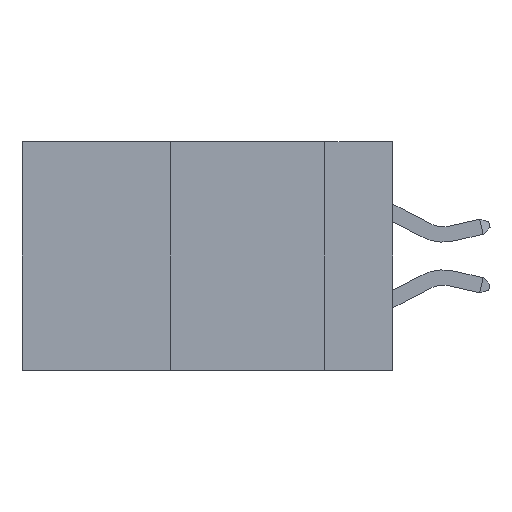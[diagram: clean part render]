
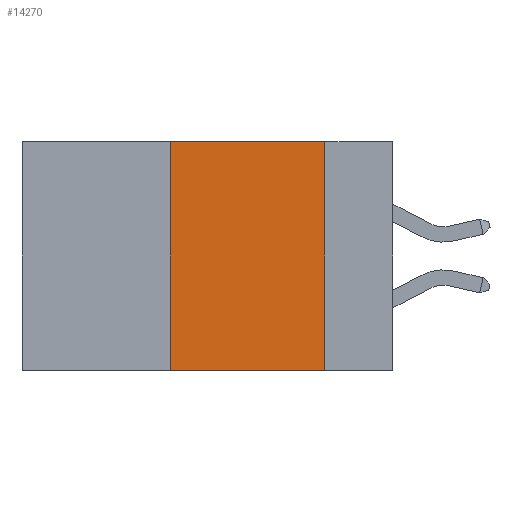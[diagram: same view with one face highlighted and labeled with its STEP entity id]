
A CAD part, left-side view. The second image highlights one B-rep face of the part: STEP entity #14270.
In plain terms, the highlighted planar face has unit normal (-1, 0, 0).
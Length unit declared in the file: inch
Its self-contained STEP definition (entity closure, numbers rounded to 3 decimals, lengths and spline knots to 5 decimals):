
#247 = VERTEX_POINT ( 'NONE', #5593 ) ;
#382 = EDGE_LOOP ( 'NONE', ( #7832, #5539, #2883, #7250 ) ) ;
#645 = EDGE_CURVE ( 'NONE', #9239, #247, #11401, .T. ) ;
#1869 = VECTOR ( 'NONE', #12145, 39.37008 ) ;
#1916 = CARTESIAN_POINT ( 'NONE',  ( 0., 0.6, 0. ) ) ;
#1929 = LINE ( 'NONE', #9311, #9542 ) ;
#2270 = VERTEX_POINT ( 'NONE', #8537 ) ;
#2870 = DIRECTION ( 'NONE',  ( 0., -1., 0. ) ) ;
#2883 = ORIENTED_EDGE ( 'NONE', *, *, #8818, .F. ) ;
#3442 = LINE ( 'NONE', #11924, #11080 ) ;
#4540 = DIRECTION ( 'NONE',  ( 0., -1., 0. ) ) ;
#4887 = CARTESIAN_POINT ( 'NONE',  ( 0., 0.11, 0. ) ) ;
#5539 = ORIENTED_EDGE ( 'NONE', *, *, #7468, .F. ) ;
#5593 = CARTESIAN_POINT ( 'NONE',  ( 0., 0.11, -0.37 ) ) ;
#6050 = AXIS2_PLACEMENT_3D ( 'NONE', #12381, #12519, #13615 ) ;
#6357 = DIRECTION ( 'NONE',  ( 0., 0., 1. ) ) ;
#6564 = CARTESIAN_POINT ( 'NONE',  ( 0., 0.11, 0. ) ) ;
#6864 = EDGE_CURVE ( 'NONE', #2270, #247, #1929, .T. ) ;
#7250 = ORIENTED_EDGE ( 'NONE', *, *, #6864, .T. ) ;
#7468 = EDGE_CURVE ( 'NONE', #9828, #9239, #9023, .T. ) ;
#7832 = ORIENTED_EDGE ( 'NONE', *, *, #645, .F. ) ;
#8537 = CARTESIAN_POINT ( 'NONE',  ( 0., 0.36, -0.37 ) ) ;
#8787 = CARTESIAN_POINT ( 'NONE',  ( 0., 0.36, 0. ) ) ;
#8818 = EDGE_CURVE ( 'NONE', #2270, #9828, #3442, .T. ) ;
#9023 = LINE ( 'NONE', #1916, #12659 ) ;
#9239 = VERTEX_POINT ( 'NONE', #4887 ) ;
#9311 = CARTESIAN_POINT ( 'NONE',  ( 0., 0.6, -0.37 ) ) ;
#9542 = VECTOR ( 'NONE', #4540, 39.37008 ) ;
#9828 = VERTEX_POINT ( 'NONE', #8787 ) ;
#10173 = PLANE ( 'NONE',  #6050 ) ;
#11080 = VECTOR ( 'NONE', #6357, 39.37008 ) ;
#11401 = LINE ( 'NONE', #6564, #1869 ) ;
#11924 = CARTESIAN_POINT ( 'NONE',  ( 0., 0.36, 0. ) ) ;
#12145 = DIRECTION ( 'NONE',  ( 0., 0., -1. ) ) ;
#12381 = CARTESIAN_POINT ( 'NONE',  ( 0., 0.6, 0. ) ) ;
#12519 = DIRECTION ( 'NONE',  ( 1., 0., 0. ) ) ;
#12659 = VECTOR ( 'NONE', #2870, 39.37008 ) ;
#13284 = FACE_OUTER_BOUND ( 'NONE', #382, .T. ) ;
#13615 = DIRECTION ( 'NONE',  ( 0., 0., -1. ) ) ;
#14270 = ADVANCED_FACE ( 'NONE', ( #13284 ), #10173, .F. ) ;
